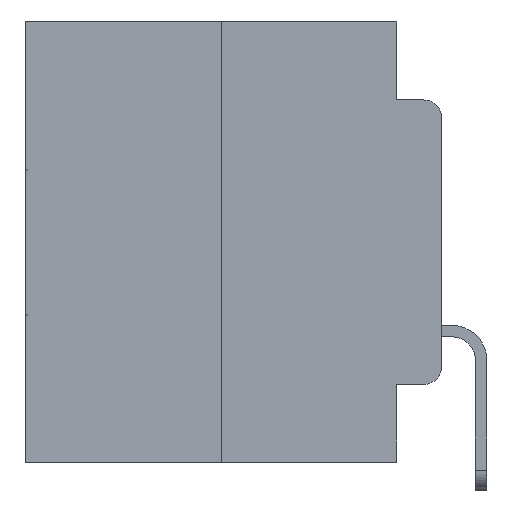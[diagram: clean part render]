
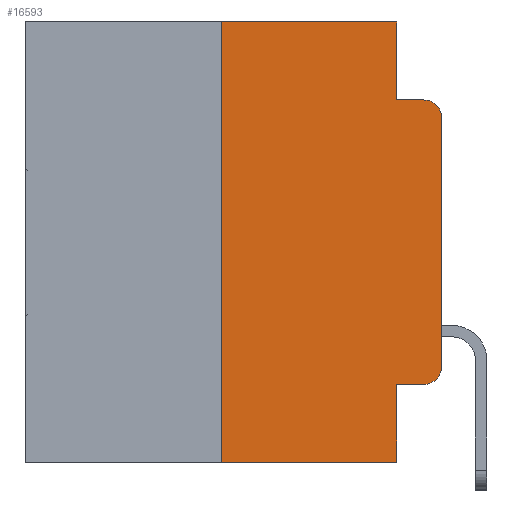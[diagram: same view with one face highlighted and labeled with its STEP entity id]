
A CAD part, left-side view. The second image highlights one B-rep face of the part: STEP entity #16593.
In plain terms, the highlighted planar face has unit normal (-1, 0, 0).
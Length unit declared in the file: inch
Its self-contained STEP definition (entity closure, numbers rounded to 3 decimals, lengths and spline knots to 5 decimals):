
#52 = CARTESIAN_POINT ( 'NONE',  ( 0., 0.051, 0. ) ) ;
#641 = VERTEX_POINT ( 'NONE', #12118 ) ;
#713 = DIRECTION ( 'NONE',  ( 0., 0., -1. ) ) ;
#2407 = ORIENTED_EDGE ( 'NONE', *, *, #6984, .F. ) ;
#2428 = DIRECTION ( 'NONE',  ( 0., 0., -1. ) ) ;
#2531 = CARTESIAN_POINT ( 'NONE',  ( 0., 0.25, -0.5 ) ) ;
#2648 = VERTEX_POINT ( 'NONE', #4452 ) ;
#3361 = EDGE_CURVE ( 'NONE', #6818, #14983, #24349, .T. ) ;
#3413 = ORIENTED_EDGE ( 'NONE', *, *, #8279, .F. ) ;
#3950 = VECTOR ( 'NONE', #11470, 39.37008 ) ;
#4452 = CARTESIAN_POINT ( 'NONE',  ( 0., 0.02, -0.4115 ) ) ;
#4759 = CARTESIAN_POINT ( 'NONE',  ( 0., 0.473, -0.5 ) ) ;
#5016 = DIRECTION ( 'NONE',  ( 0., -1., 0. ) ) ;
#5036 = DIRECTION ( 'NONE',  ( 0., 0., -1. ) ) ;
#5295 = VERTEX_POINT ( 'NONE', #14351 ) ;
#5966 = CIRCLE ( 'NONE', #25525, 0.02 ) ;
#6708 = CARTESIAN_POINT ( 'NONE',  ( 0., 0.02, -0.3915 ) ) ;
#6728 = CIRCLE ( 'NONE', #16537, 0.02 ) ;
#6818 = VERTEX_POINT ( 'NONE', #24276 ) ;
#6827 = VECTOR ( 'NONE', #12711, 39.37008 ) ;
#6965 = ORIENTED_EDGE ( 'NONE', *, *, #24592, .T. ) ;
#6984 = EDGE_CURVE ( 'NONE', #26084, #6818, #11358, .T. ) ;
#7478 = VERTEX_POINT ( 'NONE', #17556 ) ;
#7632 = VERTEX_POINT ( 'NONE', #2531 ) ;
#8279 = EDGE_CURVE ( 'NONE', #19339, #641, #28572, .T. ) ;
#8566 = VERTEX_POINT ( 'NONE', #21344 ) ;
#8589 = DIRECTION ( 'NONE',  ( 0., 0., 1. ) ) ;
#8626 = LINE ( 'NONE', #18853, #25389 ) ;
#8961 = DIRECTION ( 'NONE',  ( 0., 0., -1. ) ) ;
#10052 = VECTOR ( 'NONE', #11632, 39.37008 ) ;
#10126 = DIRECTION ( 'NONE',  ( 0., 0., 1. ) ) ;
#10995 = VECTOR ( 'NONE', #8589, 39.37008 ) ;
#11013 = ORIENTED_EDGE ( 'NONE', *, *, #19694, .T. ) ;
#11154 = FACE_OUTER_BOUND ( 'NONE', #27565, .T. ) ;
#11358 = LINE ( 'NONE', #52, #3950 ) ;
#11470 = DIRECTION ( 'NONE',  ( 0., 0., -1. ) ) ;
#11632 = DIRECTION ( 'NONE',  ( 0., -1., 0. ) ) ;
#11926 = CARTESIAN_POINT ( 'NONE',  ( 0., 0.051, -0.0885 ) ) ;
#12118 = CARTESIAN_POINT ( 'NONE',  ( 0., 0.051, -0.5 ) ) ;
#12214 = EDGE_CURVE ( 'NONE', #7478, #5295, #8626, .T. ) ;
#12711 = DIRECTION ( 'NONE',  ( 0., -1., 0. ) ) ;
#12941 = CARTESIAN_POINT ( 'NONE',  ( 0., 0.25, 0. ) ) ;
#13102 = AXIS2_PLACEMENT_3D ( 'NONE', #13528, #15833, #2428 ) ;
#13528 = CARTESIAN_POINT ( 'NONE',  ( 0., 0.473, 0. ) ) ;
#13623 = PLANE ( 'NONE',  #13102 ) ;
#14202 = DIRECTION ( 'NONE',  ( -1., 0., 0. ) ) ;
#14351 = CARTESIAN_POINT ( 'NONE',  ( 0., 0., -0.1085 ) ) ;
#14477 = CARTESIAN_POINT ( 'NONE',  ( 0., 0.02, -0.0885 ) ) ;
#14600 = ORIENTED_EDGE ( 'NONE', *, *, #3361, .F. ) ;
#14983 = VERTEX_POINT ( 'NONE', #14477 ) ;
#15833 = DIRECTION ( 'NONE',  ( 1., 0., 0. ) ) ;
#15986 = LINE ( 'NONE', #20484, #26169 ) ;
#16537 = AXIS2_PLACEMENT_3D ( 'NONE', #6708, #22099, #8961 ) ;
#16593 = ADVANCED_FACE ( 'NONE', ( #11154 ), #13623, .F. ) ;
#16606 = EDGE_CURVE ( 'NONE', #7632, #641, #28453, .T. ) ;
#17556 = CARTESIAN_POINT ( 'NONE',  ( 0., 0., -0.3915 ) ) ;
#18433 = EDGE_CURVE ( 'NONE', #8566, #26084, #21705, .T. ) ;
#18853 = CARTESIAN_POINT ( 'NONE',  ( 0., 0., 0. ) ) ;
#19339 = VERTEX_POINT ( 'NONE', #21458 ) ;
#19694 = EDGE_CURVE ( 'NONE', #19339, #2648, #15986, .T. ) ;
#19737 = ORIENTED_EDGE ( 'NONE', *, *, #18433, .F. ) ;
#20121 = ORIENTED_EDGE ( 'NONE', *, *, #16606, .T. ) ;
#20484 = CARTESIAN_POINT ( 'NONE',  ( 0., 0.051, -0.4115 ) ) ;
#20501 = CARTESIAN_POINT ( 'NONE',  ( 0., 0.051, 0. ) ) ;
#21184 = CARTESIAN_POINT ( 'NONE',  ( 0., 0.051, 0. ) ) ;
#21344 = CARTESIAN_POINT ( 'NONE',  ( 0., 0.25, 0. ) ) ;
#21458 = CARTESIAN_POINT ( 'NONE',  ( 0., 0.051, -0.4115 ) ) ;
#21705 = LINE ( 'NONE', #24704, #10052 ) ;
#22099 = DIRECTION ( 'NONE',  ( -1., 0., 0. ) ) ;
#22100 = VECTOR ( 'NONE', #22411, 39.37008 ) ;
#22155 = ORIENTED_EDGE ( 'NONE', *, *, #26225, .F. ) ;
#22411 = DIRECTION ( 'NONE',  ( 0., -1., 0. ) ) ;
#23205 = ORIENTED_EDGE ( 'NONE', *, *, #12214, .T. ) ;
#23301 = LINE ( 'NONE', #12941, #10995 ) ;
#24276 = CARTESIAN_POINT ( 'NONE',  ( 0., 0.051, -0.0885 ) ) ;
#24349 = LINE ( 'NONE', #11926, #6827 ) ;
#24498 = ORIENTED_EDGE ( 'NONE', *, *, #28358, .T. ) ;
#24592 = EDGE_CURVE ( 'NONE', #2648, #7478, #6728, .T. ) ;
#24704 = CARTESIAN_POINT ( 'NONE',  ( 0., 0.473, 0. ) ) ;
#25389 = VECTOR ( 'NONE', #10126, 39.37008 ) ;
#25525 = AXIS2_PLACEMENT_3D ( 'NONE', #27201, #14202, #713 ) ;
#26084 = VERTEX_POINT ( 'NONE', #21184 ) ;
#26169 = VECTOR ( 'NONE', #5016, 39.37008 ) ;
#26225 = EDGE_CURVE ( 'NONE', #7632, #8566, #23301, .T. ) ;
#27201 = CARTESIAN_POINT ( 'NONE',  ( 0., 0.02, -0.1085 ) ) ;
#27253 = VECTOR ( 'NONE', #5036, 39.37008 ) ;
#27565 = EDGE_LOOP ( 'NONE', ( #23205, #24498, #14600, #2407, #19737, #22155, #20121, #3413, #11013, #6965 ) ) ;
#28358 = EDGE_CURVE ( 'NONE', #5295, #14983, #5966, .T. ) ;
#28453 = LINE ( 'NONE', #4759, #22100 ) ;
#28572 = LINE ( 'NONE', #20501, #27253 ) ;
